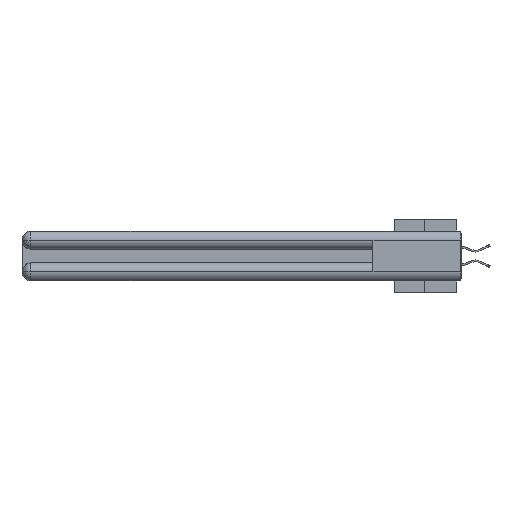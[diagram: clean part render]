
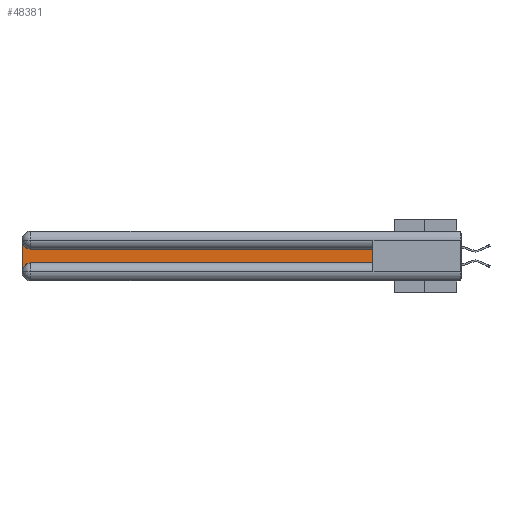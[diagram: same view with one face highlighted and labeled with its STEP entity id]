
A CAD part, left-side view. The second image highlights one B-rep face of the part: STEP entity #48381.
In plain terms, the highlighted planar face has unit normal (-1, 0, 0).
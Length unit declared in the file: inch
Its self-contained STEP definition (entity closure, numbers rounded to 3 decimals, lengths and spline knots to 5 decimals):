
#82 = CIRCLE ( 'NONE', #520, 0.06 ) ;
#520 = AXIS2_PLACEMENT_3D ( 'NONE', #47316, #8225, #28518 ) ;
#2536 = CARTESIAN_POINT ( 'NONE',  ( 0.075, 3., -0.2775 ) ) ;
#4381 = EDGE_CURVE ( 'NONE', #14065, #14605, #82, .T. ) ;
#4409 = LINE ( 'NONE', #32166, #38906 ) ;
#6613 = ORIENTED_EDGE ( 'NONE', *, *, #31191, .T. ) ;
#6827 = DIRECTION ( 'NONE',  ( 0., 0., -1. ) ) ;
#7162 = CARTESIAN_POINT ( 'NONE',  ( 0.075, 3., -0.1225 ) ) ;
#7351 = VERTEX_POINT ( 'NONE', #47741 ) ;
#7804 = CARTESIAN_POINT ( 'NONE',  ( 0.075, 2.94, -0.2175 ) ) ;
#8225 = DIRECTION ( 'NONE',  ( 1., 0., 0. ) ) ;
#12423 = ORIENTED_EDGE ( 'NONE', *, *, #30522, .T. ) ;
#14065 = VERTEX_POINT ( 'NONE', #2536 ) ;
#14428 = CARTESIAN_POINT ( 'NONE',  ( 0.075, 0.6, -0.2175 ) ) ;
#14565 = LINE ( 'NONE', #45242, #39614 ) ;
#14578 = CARTESIAN_POINT ( 'NONE',  ( 0.075, 0.6, -0.2175 ) ) ;
#14605 = VERTEX_POINT ( 'NONE', #7804 ) ;
#16018 = ORIENTED_EDGE ( 'NONE', *, *, #24400, .T. ) ;
#18050 = FACE_OUTER_BOUND ( 'NONE', #23511, .T. ) ;
#19423 = DIRECTION ( 'NONE',  ( 0., 0., -1. ) ) ;
#19573 = CARTESIAN_POINT ( 'NONE',  ( 0.075, 0.6, -0.2175 ) ) ;
#20088 = ORIENTED_EDGE ( 'NONE', *, *, #32204, .T. ) ;
#20277 = LINE ( 'NONE', #14428, #45879 ) ;
#23511 = EDGE_LOOP ( 'NONE', ( #16018, #12423, #39858, #35558, #20088, #6613 ) ) ;
#24400 = EDGE_CURVE ( 'NONE', #31312, #7351, #4409, .T. ) ;
#26105 = VECTOR ( 'NONE', #45438, 39.37008 ) ;
#27677 = EDGE_CURVE ( 'NONE', #35289, #14065, #14565, .T. ) ;
#28518 = DIRECTION ( 'NONE',  ( 0., 0., -1. ) ) ;
#29431 = CARTESIAN_POINT ( 'NONE',  ( 0.075, 2.94, -0.0625 ) ) ;
#30522 = EDGE_CURVE ( 'NONE', #7351, #35289, #46541, .T. ) ;
#31051 = AXIS2_PLACEMENT_3D ( 'NONE', #7162, #45288, #34090 ) ;
#31191 = EDGE_CURVE ( 'NONE', #47147, #31312, #20277, .T. ) ;
#31218 = AXIS2_PLACEMENT_3D ( 'NONE', #29431, #44779, #6827 ) ;
#31312 = VERTEX_POINT ( 'NONE', #42577 ) ;
#32166 = CARTESIAN_POINT ( 'NONE',  ( 0.075, 0.6, -0.1225 ) ) ;
#32204 = EDGE_CURVE ( 'NONE', #14605, #47147, #35607, .T. ) ;
#33428 = DIRECTION ( 'NONE',  ( 0., 0., 1. ) ) ;
#34090 = DIRECTION ( 'NONE',  ( 0., 0., -1. ) ) ;
#35289 = VERTEX_POINT ( 'NONE', #37664 ) ;
#35558 = ORIENTED_EDGE ( 'NONE', *, *, #4381, .T. ) ;
#35607 = LINE ( 'NONE', #14578, #26105 ) ;
#37267 = PLANE ( 'NONE',  #31051 ) ;
#37664 = CARTESIAN_POINT ( 'NONE',  ( 0.075, 3., -0.0625 ) ) ;
#38906 = VECTOR ( 'NONE', #47161, 39.37008 ) ;
#39614 = VECTOR ( 'NONE', #19423, 39.37008 ) ;
#39858 = ORIENTED_EDGE ( 'NONE', *, *, #27677, .T. ) ;
#42577 = CARTESIAN_POINT ( 'NONE',  ( 0.075, 0.6, -0.1225 ) ) ;
#44779 = DIRECTION ( 'NONE',  ( 1., 0., 0. ) ) ;
#45242 = CARTESIAN_POINT ( 'NONE',  ( 0.075, 3., -0.2175 ) ) ;
#45288 = DIRECTION ( 'NONE',  ( 1., 0., 0. ) ) ;
#45438 = DIRECTION ( 'NONE',  ( 0., -1., 0. ) ) ;
#45879 = VECTOR ( 'NONE', #33428, 39.37008 ) ;
#46541 = CIRCLE ( 'NONE', #31218, 0.06 ) ;
#47147 = VERTEX_POINT ( 'NONE', #19573 ) ;
#47161 = DIRECTION ( 'NONE',  ( 0., 1., 0. ) ) ;
#47316 = CARTESIAN_POINT ( 'NONE',  ( 0.075, 2.94, -0.2775 ) ) ;
#47741 = CARTESIAN_POINT ( 'NONE',  ( 0.075, 2.94, -0.1225 ) ) ;
#48381 = ADVANCED_FACE ( 'NONE', ( #18050 ), #37267, .F. ) ;
